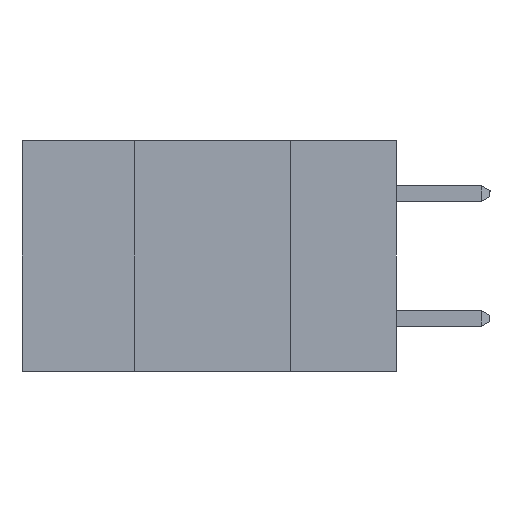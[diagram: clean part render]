
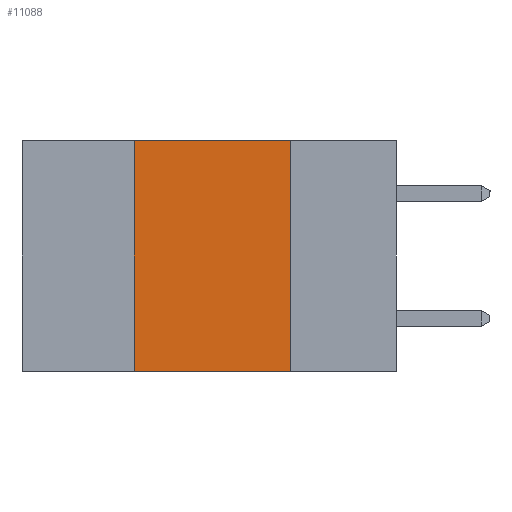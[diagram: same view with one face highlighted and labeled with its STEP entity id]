
A CAD part, left-side view. The second image highlights one B-rep face of the part: STEP entity #11088.
In plain terms, the highlighted planar face has unit normal (-1, 0, 0).
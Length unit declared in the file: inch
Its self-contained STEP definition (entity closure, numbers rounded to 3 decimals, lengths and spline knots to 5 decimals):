
#23 = CARTESIAN_POINT ( 'NONE',  ( 0., 0.6, -0.37 ) ) ;
#589 = CARTESIAN_POINT ( 'NONE',  ( 0., 0.42, -0.37 ) ) ;
#724 = ORIENTED_EDGE ( 'NONE', *, *, #2141, .F. ) ;
#1030 = AXIS2_PLACEMENT_3D ( 'NONE', #9384, #6178, #2693 ) ;
#1200 = VERTEX_POINT ( 'NONE', #5936 ) ;
#1482 = CARTESIAN_POINT ( 'NONE',  ( 0., 0.17, -0.37 ) ) ;
#1526 = CARTESIAN_POINT ( 'NONE',  ( 0., 0.17, 0. ) ) ;
#2141 = EDGE_CURVE ( 'NONE', #1200, #11836, #4973, .T. ) ;
#2241 = LINE ( 'NONE', #10378, #2882 ) ;
#2289 = DIRECTION ( 'NONE',  ( 0., 0., -1. ) ) ;
#2693 = DIRECTION ( 'NONE',  ( 0., 0., -1. ) ) ;
#2882 = VECTOR ( 'NONE', #5706, 39.37008 ) ;
#3065 = EDGE_CURVE ( 'NONE', #10702, #14424, #3718, .T. ) ;
#3400 = DIRECTION ( 'NONE',  ( 0., -1., 0. ) ) ;
#3498 = EDGE_CURVE ( 'NONE', #1200, #14424, #4615, .T. ) ;
#3718 = LINE ( 'NONE', #8304, #8945 ) ;
#4615 = LINE ( 'NONE', #23, #5401 ) ;
#4719 = ORIENTED_EDGE ( 'NONE', *, *, #3065, .F. ) ;
#4819 = FACE_OUTER_BOUND ( 'NONE', #14647, .T. ) ;
#4973 = LINE ( 'NONE', #589, #5303 ) ;
#5303 = VECTOR ( 'NONE', #10612, 39.37008 ) ;
#5336 = ORIENTED_EDGE ( 'NONE', *, *, #3498, .T. ) ;
#5401 = VECTOR ( 'NONE', #3400, 39.37008 ) ;
#5706 = DIRECTION ( 'NONE',  ( 0., -1., 0. ) ) ;
#5936 = CARTESIAN_POINT ( 'NONE',  ( 0., 0.42, -0.37 ) ) ;
#6178 = DIRECTION ( 'NONE',  ( 1., 0., 0. ) ) ;
#6857 = EDGE_CURVE ( 'NONE', #11836, #10702, #2241, .T. ) ;
#8304 = CARTESIAN_POINT ( 'NONE',  ( 0., 0.17, -0.37 ) ) ;
#8404 = PLANE ( 'NONE',  #1030 ) ;
#8945 = VECTOR ( 'NONE', #2289, 39.37008 ) ;
#9384 = CARTESIAN_POINT ( 'NONE',  ( 0., 0.6, 0. ) ) ;
#9445 = ORIENTED_EDGE ( 'NONE', *, *, #6857, .F. ) ;
#10378 = CARTESIAN_POINT ( 'NONE',  ( 0., 0.6, 0. ) ) ;
#10612 = DIRECTION ( 'NONE',  ( 0., 0., 1. ) ) ;
#10702 = VERTEX_POINT ( 'NONE', #1526 ) ;
#10945 = CARTESIAN_POINT ( 'NONE',  ( 0., 0.42, 0. ) ) ;
#11088 = ADVANCED_FACE ( 'NONE', ( #4819 ), #8404, .F. ) ;
#11836 = VERTEX_POINT ( 'NONE', #10945 ) ;
#14424 = VERTEX_POINT ( 'NONE', #1482 ) ;
#14647 = EDGE_LOOP ( 'NONE', ( #4719, #9445, #724, #5336 ) ) ;
